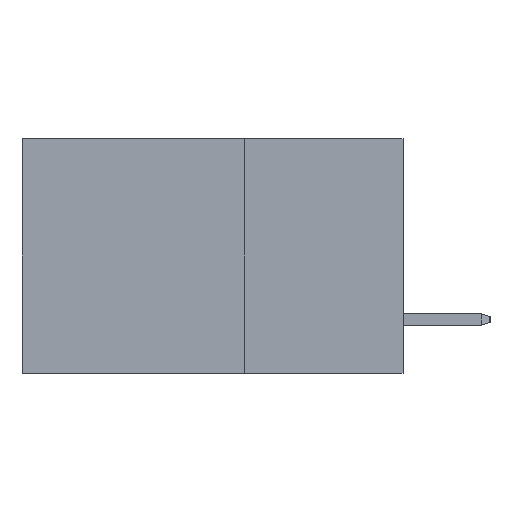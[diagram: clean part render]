
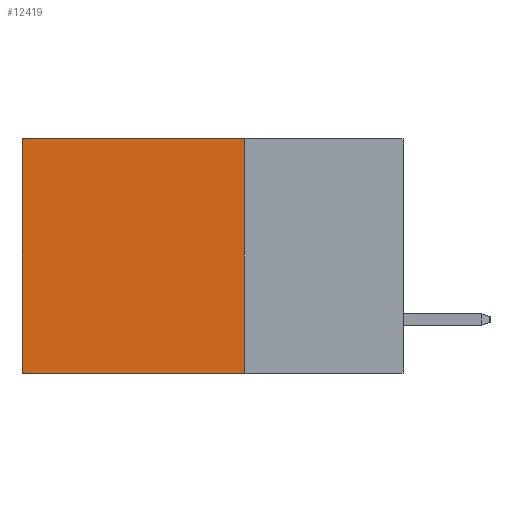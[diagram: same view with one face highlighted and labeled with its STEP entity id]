
A CAD part, left-side view. The second image highlights one B-rep face of the part: STEP entity #12419.
In plain terms, the highlighted planar face has unit normal (-1, 0, 0).
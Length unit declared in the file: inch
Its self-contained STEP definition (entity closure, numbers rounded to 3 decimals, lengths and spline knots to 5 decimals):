
#6 = EDGE_LOOP ( 'NONE', ( #24876, #19277, #12255, #3934 ) ) ;
#1367 = DIRECTION ( 'NONE',  ( 0., 0., -1. ) ) ;
#2096 = CARTESIAN_POINT ( 'NONE',  ( 0.2875, 0.25, -0.37 ) ) ;
#3478 = CARTESIAN_POINT ( 'NONE',  ( 0.2875, 0.25, 0. ) ) ;
#3535 = CARTESIAN_POINT ( 'NONE',  ( 0.2875, 0.6, 0. ) ) ;
#3934 = ORIENTED_EDGE ( 'NONE', *, *, #14765, .T. ) ;
#4470 = VERTEX_POINT ( 'NONE', #21140 ) ;
#5117 = DIRECTION ( 'NONE',  ( 0., 0., -1. ) ) ;
#5752 = DIRECTION ( 'NONE',  ( 0., 0., -1. ) ) ;
#7359 = VERTEX_POINT ( 'NONE', #17663 ) ;
#7489 = LINE ( 'NONE', #3535, #25396 ) ;
#7761 = EDGE_CURVE ( 'NONE', #22641, #8198, #17499, .T. ) ;
#8161 = DIRECTION ( 'NONE',  ( 0., 1., 0. ) ) ;
#8198 = VERTEX_POINT ( 'NONE', #19718 ) ;
#9557 = FACE_OUTER_BOUND ( 'NONE', #6, .T. ) ;
#10280 = EDGE_CURVE ( 'NONE', #7359, #4470, #7489, .T. ) ;
#11271 = DIRECTION ( 'NONE',  ( 0., 1., 0. ) ) ;
#12255 = ORIENTED_EDGE ( 'NONE', *, *, #7761, .F. ) ;
#12419 = ADVANCED_FACE ( 'NONE', ( #9557 ), #17608, .F. ) ;
#14765 = EDGE_CURVE ( 'NONE', #22641, #7359, #24758, .T. ) ;
#17213 = CARTESIAN_POINT ( 'NONE',  ( 0.2875, 0.25, 0. ) ) ;
#17499 = LINE ( 'NONE', #23959, #22838 ) ;
#17608 = PLANE ( 'NONE',  #25061 ) ;
#17663 = CARTESIAN_POINT ( 'NONE',  ( 0.2875, 0.6, 0. ) ) ;
#18073 = LINE ( 'NONE', #2096, #23533 ) ;
#19277 = ORIENTED_EDGE ( 'NONE', *, *, #25580, .F. ) ;
#19718 = CARTESIAN_POINT ( 'NONE',  ( 0.2875, 0.25, -0.37 ) ) ;
#20679 = CARTESIAN_POINT ( 'NONE',  ( 0.2875, 0.25, 0. ) ) ;
#21140 = CARTESIAN_POINT ( 'NONE',  ( 0.2875, 0.6, -0.37 ) ) ;
#22641 = VERTEX_POINT ( 'NONE', #17213 ) ;
#22838 = VECTOR ( 'NONE', #5752, 39.37008 ) ;
#23533 = VECTOR ( 'NONE', #8161, 39.37008 ) ;
#23959 = CARTESIAN_POINT ( 'NONE',  ( 0.2875, 0.25, 0. ) ) ;
#24758 = LINE ( 'NONE', #20679, #26003 ) ;
#24876 = ORIENTED_EDGE ( 'NONE', *, *, #10280, .T. ) ;
#25061 = AXIS2_PLACEMENT_3D ( 'NONE', #3478, #25263, #1367 ) ;
#25263 = DIRECTION ( 'NONE',  ( 1., 0., 0. ) ) ;
#25396 = VECTOR ( 'NONE', #5117, 39.37008 ) ;
#25580 = EDGE_CURVE ( 'NONE', #8198, #4470, #18073, .T. ) ;
#26003 = VECTOR ( 'NONE', #11271, 39.37008 ) ;
